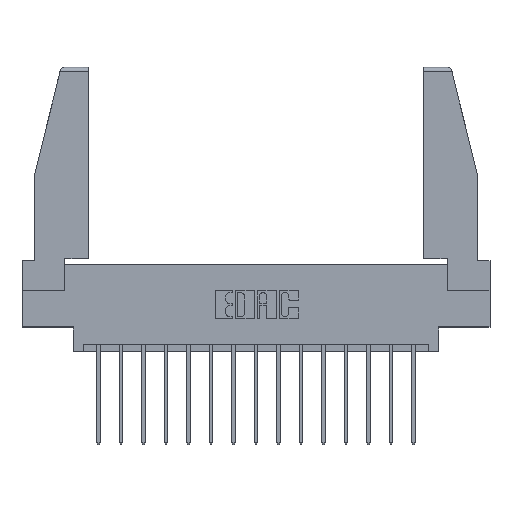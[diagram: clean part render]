
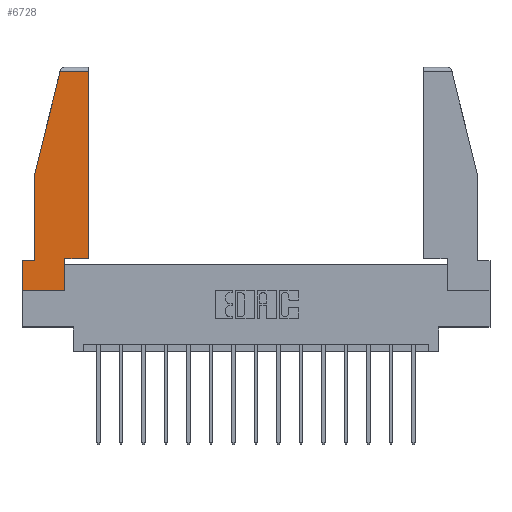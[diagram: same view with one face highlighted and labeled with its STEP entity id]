
A CAD part, top view. The second image highlights one B-rep face of the part: STEP entity #6728.
In plain terms, the highlighted planar face has unit normal (0, 0, 1).
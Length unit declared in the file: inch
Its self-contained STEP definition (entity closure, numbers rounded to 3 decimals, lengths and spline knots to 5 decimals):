
#491 = CARTESIAN_POINT ( 'NONE',  ( 0., 0., 0. ) ) ;
#784 = DIRECTION ( 'NONE',  ( 0., 0., 1. ) ) ;
#818 = ORIENTED_EDGE ( 'NONE', *, *, #6382, .T. ) ;
#1167 = LINE ( 'NONE', #5484, #15772 ) ;
#1454 = VERTEX_POINT ( 'NONE', #16928 ) ;
#1697 = ORIENTED_EDGE ( 'NONE', *, *, #2560, .T. ) ;
#1733 = ORIENTED_EDGE ( 'NONE', *, *, #7007, .T. ) ;
#1814 = VERTEX_POINT ( 'NONE', #13644 ) ;
#2204 = CARTESIAN_POINT ( 'NONE',  ( 0.297, 0.223, 0. ) ) ;
#2425 = CARTESIAN_POINT ( 'NONE',  ( 0.086, 0.21, 0. ) ) ;
#2476 = VECTOR ( 'NONE', #4186, 39.37008 ) ;
#2560 = EDGE_CURVE ( 'NONE', #8169, #1814, #14214, .T. ) ;
#2617 = DIRECTION ( 'NONE',  ( 0., -1., 0. ) ) ;
#2676 = VERTEX_POINT ( 'NONE', #2425 ) ;
#2811 = CARTESIAN_POINT ( 'NONE',  ( 0., 0., 0. ) ) ;
#2873 = LINE ( 'NONE', #4734, #7166 ) ;
#3294 = VERTEX_POINT ( 'NONE', #17267 ) ;
#3468 = DIRECTION ( 'NONE',  ( -1., 0., 0. ) ) ;
#3483 = LINE ( 'NONE', #13437, #10357 ) ;
#4186 = DIRECTION ( 'NONE',  ( 1., 0., 0. ) ) ;
#4324 = EDGE_LOOP ( 'NONE', ( #7270, #8249, #9761, #7536, #818, #1733, #9047, #1697, #14927 ) ) ;
#4734 = CARTESIAN_POINT ( 'NONE',  ( 0., 0.21, 0. ) ) ;
#4770 = CARTESIAN_POINT ( 'NONE',  ( 0.086, 0.8, 0. ) ) ;
#5249 = CARTESIAN_POINT ( 'NONE',  ( 0.086, 0.8, 0. ) ) ;
#5304 = LINE ( 'NONE', #17148, #11764 ) ;
#5484 = CARTESIAN_POINT ( 'NONE',  ( 0.461, 0.223, 0. ) ) ;
#5504 = EDGE_CURVE ( 'NONE', #1454, #3294, #17067, .T. ) ;
#5670 = EDGE_CURVE ( 'NONE', #17041, #8169, #14094, .T. ) ;
#6126 = DIRECTION ( 'NONE',  ( -0.239, -0.971, 0. ) ) ;
#6283 = LINE ( 'NONE', #2204, #11878 ) ;
#6382 = EDGE_CURVE ( 'NONE', #2676, #11230, #2873, .T. ) ;
#6728 = ADVANCED_FACE ( 'NONE', ( #16395 ), #11772, .T. ) ;
#7007 = EDGE_CURVE ( 'NONE', #11230, #17041, #3483, .T. ) ;
#7166 = VECTOR ( 'NONE', #3468, 39.37008 ) ;
#7270 = ORIENTED_EDGE ( 'NONE', *, *, #9872, .T. ) ;
#7291 = VECTOR ( 'NONE', #11740, 39.37008 ) ;
#7536 = ORIENTED_EDGE ( 'NONE', *, *, #8719, .T. ) ;
#8169 = VERTEX_POINT ( 'NONE', #14232 ) ;
#8249 = ORIENTED_EDGE ( 'NONE', *, *, #5504, .T. ) ;
#8344 = AXIS2_PLACEMENT_3D ( 'NONE', #13216, #784, #15960 ) ;
#8719 = EDGE_CURVE ( 'NONE', #13783, #2676, #12179, .T. ) ;
#9047 = ORIENTED_EDGE ( 'NONE', *, *, #5670, .T. ) ;
#9761 = ORIENTED_EDGE ( 'NONE', *, *, #13898, .T. ) ;
#9872 = EDGE_CURVE ( 'NONE', #11965, #1454, #1167, .T. ) ;
#10357 = VECTOR ( 'NONE', #2617, 39.37008 ) ;
#10692 = CARTESIAN_POINT ( 'NONE',  ( 0., 1.52, 0. ) ) ;
#10712 = EDGE_CURVE ( 'NONE', #1814, #11965, #6283, .T. ) ;
#11118 = CARTESIAN_POINT ( 'NONE',  ( 0.461, 0.223, 0. ) ) ;
#11230 = VERTEX_POINT ( 'NONE', #16479 ) ;
#11740 = DIRECTION ( 'NONE',  ( 0., 1., 0. ) ) ;
#11764 = VECTOR ( 'NONE', #6126, 39.37008 ) ;
#11772 = PLANE ( 'NONE',  #8344 ) ;
#11878 = VECTOR ( 'NONE', #17544, 39.37008 ) ;
#11965 = VERTEX_POINT ( 'NONE', #11118 ) ;
#12179 = LINE ( 'NONE', #4770, #15398 ) ;
#13216 = CARTESIAN_POINT ( 'NONE',  ( 0., 0., 0. ) ) ;
#13238 = CARTESIAN_POINT ( 'NONE',  ( 0.297, 0., 0. ) ) ;
#13437 = CARTESIAN_POINT ( 'NONE',  ( 0., 0.21, 0. ) ) ;
#13644 = CARTESIAN_POINT ( 'NONE',  ( 0.297, 0.223, 0. ) ) ;
#13783 = VERTEX_POINT ( 'NONE', #5249 ) ;
#13898 = EDGE_CURVE ( 'NONE', #3294, #13783, #5304, .T. ) ;
#14094 = LINE ( 'NONE', #2811, #2476 ) ;
#14214 = LINE ( 'NONE', #13238, #7291 ) ;
#14232 = CARTESIAN_POINT ( 'NONE',  ( 0.297, 0., 0. ) ) ;
#14927 = ORIENTED_EDGE ( 'NONE', *, *, #10712, .T. ) ;
#15108 = DIRECTION ( 'NONE',  ( 0., 1., 0. ) ) ;
#15398 = VECTOR ( 'NONE', #15940, 39.37008 ) ;
#15772 = VECTOR ( 'NONE', #15108, 39.37008 ) ;
#15940 = DIRECTION ( 'NONE',  ( 0., -1., 0. ) ) ;
#15960 = DIRECTION ( 'NONE',  ( 1., 0., 0. ) ) ;
#16395 = FACE_OUTER_BOUND ( 'NONE', #4324, .T. ) ;
#16479 = CARTESIAN_POINT ( 'NONE',  ( 0., 0.21, 0. ) ) ;
#16928 = CARTESIAN_POINT ( 'NONE',  ( 0.461, 1.52, 0. ) ) ;
#17041 = VERTEX_POINT ( 'NONE', #491 ) ;
#17067 = LINE ( 'NONE', #10692, #17693 ) ;
#17148 = CARTESIAN_POINT ( 'NONE',  ( 0.271, 1.55, 0. ) ) ;
#17267 = CARTESIAN_POINT ( 'NONE',  ( 0.2636, 1.52, 0. ) ) ;
#17544 = DIRECTION ( 'NONE',  ( 1., 0., 0. ) ) ;
#17610 = DIRECTION ( 'NONE',  ( -1., 0., 0. ) ) ;
#17693 = VECTOR ( 'NONE', #17610, 39.37008 ) ;
